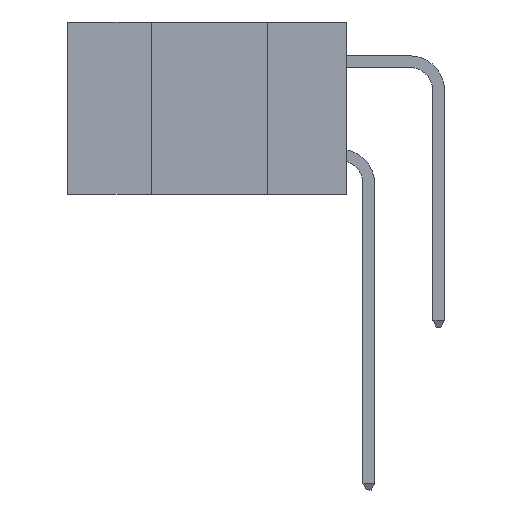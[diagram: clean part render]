
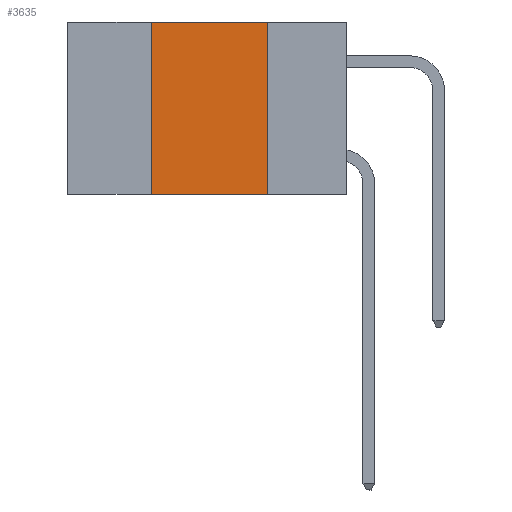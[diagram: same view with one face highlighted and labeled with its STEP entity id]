
A CAD part, left-side view. The second image highlights one B-rep face of the part: STEP entity #3635.
In plain terms, the highlighted planar face has unit normal (-1, 0, 0).
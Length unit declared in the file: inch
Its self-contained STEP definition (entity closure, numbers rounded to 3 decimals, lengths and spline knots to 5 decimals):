
#1651 = VERTEX_POINT ( 'NONE', #1952 ) ;
#1694 = ORIENTED_EDGE ( 'NONE', *, *, #11032, .F. ) ;
#1952 = CARTESIAN_POINT ( 'NONE',  ( 0., 0.17, 0. ) ) ;
#2201 = PLANE ( 'NONE',  #10404 ) ;
#2628 = DIRECTION ( 'NONE',  ( 0., 0., 1. ) ) ;
#2853 = LINE ( 'NONE', #4955, #6868 ) ;
#3635 = ADVANCED_FACE ( 'NONE', ( #13244 ), #2201, .F. ) ;
#4040 = VECTOR ( 'NONE', #2628, 39.37008 ) ;
#4343 = EDGE_CURVE ( 'NONE', #11175, #1651, #12048, .T. ) ;
#4347 = DIRECTION ( 'NONE',  ( 0., -1., 0. ) ) ;
#4588 = LINE ( 'NONE', #9013, #4040 ) ;
#4597 = DIRECTION ( 'NONE',  ( 1., 0., 0. ) ) ;
#4820 = CARTESIAN_POINT ( 'NONE',  ( 0., 0.6, -0.37 ) ) ;
#4955 = CARTESIAN_POINT ( 'NONE',  ( 0., 0.17, 0. ) ) ;
#5074 = CARTESIAN_POINT ( 'NONE',  ( 0., 0.42, -0.37 ) ) ;
#5296 = CARTESIAN_POINT ( 'NONE',  ( 0., 0.42, 0. ) ) ;
#6622 = CARTESIAN_POINT ( 'NONE',  ( 0., 0.6, 0. ) ) ;
#6868 = VECTOR ( 'NONE', #8215, 39.37008 ) ;
#8215 = DIRECTION ( 'NONE',  ( 0., 0., -1. ) ) ;
#8829 = VECTOR ( 'NONE', #4347, 39.37008 ) ;
#9013 = CARTESIAN_POINT ( 'NONE',  ( 0., 0.42, 0. ) ) ;
#9189 = ORIENTED_EDGE ( 'NONE', *, *, #9360, .T. ) ;
#9210 = EDGE_LOOP ( 'NONE', ( #12191, #11908, #1694, #9189 ) ) ;
#9247 = DIRECTION ( 'NONE',  ( 0., -1., 0. ) ) ;
#9360 = EDGE_CURVE ( 'NONE', #12583, #11548, #12454, .T. ) ;
#10404 = AXIS2_PLACEMENT_3D ( 'NONE', #6622, #4597, #10406 ) ;
#10406 = DIRECTION ( 'NONE',  ( 0., 0., -1. ) ) ;
#10810 = CARTESIAN_POINT ( 'NONE',  ( 0., 0.6, 0. ) ) ;
#11032 = EDGE_CURVE ( 'NONE', #12583, #11175, #4588, .T. ) ;
#11175 = VERTEX_POINT ( 'NONE', #5296 ) ;
#11260 = CARTESIAN_POINT ( 'NONE',  ( 0., 0.17, -0.37 ) ) ;
#11548 = VERTEX_POINT ( 'NONE', #11260 ) ;
#11908 = ORIENTED_EDGE ( 'NONE', *, *, #4343, .F. ) ;
#12048 = LINE ( 'NONE', #10810, #8829 ) ;
#12191 = ORIENTED_EDGE ( 'NONE', *, *, #13451, .F. ) ;
#12454 = LINE ( 'NONE', #4820, #13496 ) ;
#12583 = VERTEX_POINT ( 'NONE', #5074 ) ;
#13244 = FACE_OUTER_BOUND ( 'NONE', #9210, .T. ) ;
#13451 = EDGE_CURVE ( 'NONE', #1651, #11548, #2853, .T. ) ;
#13496 = VECTOR ( 'NONE', #9247, 39.37008 ) ;
